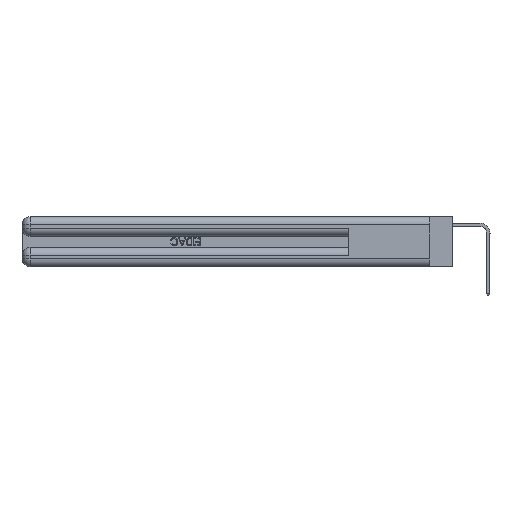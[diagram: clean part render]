
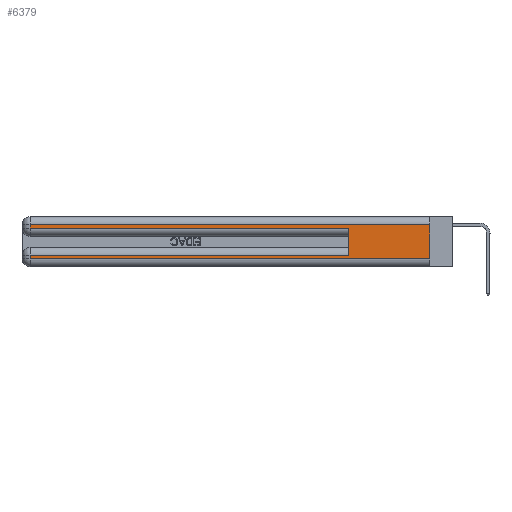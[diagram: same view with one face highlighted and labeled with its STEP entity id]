
A CAD part, left-side view. The second image highlights one B-rep face of the part: STEP entity #6379.
In plain terms, the highlighted planar face has unit normal (-1, 0, 0).
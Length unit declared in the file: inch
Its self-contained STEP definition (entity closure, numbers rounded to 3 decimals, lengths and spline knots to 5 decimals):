
#803 = CARTESIAN_POINT ( 'NONE',  ( 0., 0., 0.06 ) ) ;
#1108 = DIRECTION ( 'NONE',  ( 1., 0., 0. ) ) ;
#1264 = ORIENTED_EDGE ( 'NONE', *, *, #27751, .T. ) ;
#1280 = CARTESIAN_POINT ( 'NONE',  ( 0., 0., 0.085 ) ) ;
#1477 = CARTESIAN_POINT ( 'NONE',  ( 0., 0., 0.31 ) ) ;
#1805 = VERTEX_POINT ( 'NONE', #10659 ) ;
#2046 = VECTOR ( 'NONE', #2947, 39.37008 ) ;
#2652 = VECTOR ( 'NONE', #3811, 39.37008 ) ;
#2755 = EDGE_CURVE ( 'NONE', #1805, #22360, #28790, .T. ) ;
#2947 = DIRECTION ( 'NONE',  ( 0., -1., 0. ) ) ;
#3811 = DIRECTION ( 'NONE',  ( 0., 1., 0. ) ) ;
#4373 = ORIENTED_EDGE ( 'NONE', *, *, #18867, .F. ) ;
#4501 = ORIENTED_EDGE ( 'NONE', *, *, #19340, .T. ) ;
#4891 = DIRECTION ( 'NONE',  ( 0., 0., -1. ) ) ;
#5882 = LINE ( 'NONE', #19683, #18463 ) ;
#6379 = ADVANCED_FACE ( 'NONE', ( #28325 ), #21110, .F. ) ;
#6913 = ORIENTED_EDGE ( 'NONE', *, *, #18565, .T. ) ;
#7429 = CARTESIAN_POINT ( 'NONE',  ( 0., 2.94, 0.37 ) ) ;
#7513 = VECTOR ( 'NONE', #14542, 39.37008 ) ;
#7570 = ORIENTED_EDGE ( 'NONE', *, *, #12561, .F. ) ;
#8049 = VECTOR ( 'NONE', #4891, 39.37008 ) ;
#9258 = CARTESIAN_POINT ( 'NONE',  ( 0., 0.6, 0.085 ) ) ;
#9781 = EDGE_CURVE ( 'NONE', #11897, #27808, #30049, .T. ) ;
#10478 = DIRECTION ( 'NONE',  ( 0., 0., -1. ) ) ;
#10659 = CARTESIAN_POINT ( 'NONE',  ( 0., 2.94, 0.085 ) ) ;
#11897 = VERTEX_POINT ( 'NONE', #15726 ) ;
#12457 = VERTEX_POINT ( 'NONE', #9258 ) ;
#12561 = EDGE_CURVE ( 'NONE', #19216, #31814, #5882, .T. ) ;
#14406 = VECTOR ( 'NONE', #10478, 39.37008 ) ;
#14542 = DIRECTION ( 'NONE',  ( 0., 1., 0. ) ) ;
#14959 = LINE ( 'NONE', #24525, #7513 ) ;
#15470 = CARTESIAN_POINT ( 'NONE',  ( 0., 0., 0.06 ) ) ;
#15726 = CARTESIAN_POINT ( 'NONE',  ( 0., 2.94, 0.285 ) ) ;
#15993 = CARTESIAN_POINT ( 'NONE',  ( 0., 2.94, 0.06 ) ) ;
#17587 = VECTOR ( 'NONE', #32317, 39.37008 ) ;
#18463 = VECTOR ( 'NONE', #22222, 39.37008 ) ;
#18565 = EDGE_CURVE ( 'NONE', #22360, #31814, #22096, .T. ) ;
#18676 = DIRECTION ( 'NONE',  ( 0., 0., -1. ) ) ;
#18867 = EDGE_CURVE ( 'NONE', #12457, #27808, #26753, .T. ) ;
#19216 = VERTEX_POINT ( 'NONE', #1477 ) ;
#19340 = EDGE_CURVE ( 'NONE', #19216, #24897, #14959, .T. ) ;
#19683 = CARTESIAN_POINT ( 'NONE',  ( 0., 0., 0.37 ) ) ;
#21110 = PLANE ( 'NONE',  #25743 ) ;
#22096 = LINE ( 'NONE', #15470, #2046 ) ;
#22222 = DIRECTION ( 'NONE',  ( 0., 0., -1. ) ) ;
#22360 = VERTEX_POINT ( 'NONE', #15993 ) ;
#22440 = EDGE_LOOP ( 'NONE', ( #7570, #4501, #1264, #24228, #4373, #30800, #30573, #6913 ) ) ;
#22497 = DIRECTION ( 'NONE',  ( 0., 0., 1. ) ) ;
#22991 = CARTESIAN_POINT ( 'NONE',  ( 0., 2.94, 0.37 ) ) ;
#24228 = ORIENTED_EDGE ( 'NONE', *, *, #9781, .T. ) ;
#24525 = CARTESIAN_POINT ( 'NONE',  ( 0., 0., 0.31 ) ) ;
#24861 = CARTESIAN_POINT ( 'NONE',  ( 0., 0., 0.285 ) ) ;
#24897 = VERTEX_POINT ( 'NONE', #28374 ) ;
#25608 = CARTESIAN_POINT ( 'NONE',  ( 0., 0.6, 0.285 ) ) ;
#25743 = AXIS2_PLACEMENT_3D ( 'NONE', #31086, #1108, #18676 ) ;
#25965 = VECTOR ( 'NONE', #22497, 39.37008 ) ;
#26753 = LINE ( 'NONE', #29857, #25965 ) ;
#27751 = EDGE_CURVE ( 'NONE', #24897, #11897, #28472, .T. ) ;
#27808 = VERTEX_POINT ( 'NONE', #25608 ) ;
#28325 = FACE_OUTER_BOUND ( 'NONE', #22440, .T. ) ;
#28374 = CARTESIAN_POINT ( 'NONE',  ( 0., 2.94, 0.31 ) ) ;
#28472 = LINE ( 'NONE', #22991, #14406 ) ;
#28790 = LINE ( 'NONE', #7429, #8049 ) ;
#29261 = LINE ( 'NONE', #1280, #2652 ) ;
#29857 = CARTESIAN_POINT ( 'NONE',  ( 0., 0.6, 0.145 ) ) ;
#30049 = LINE ( 'NONE', #24861, #17587 ) ;
#30573 = ORIENTED_EDGE ( 'NONE', *, *, #2755, .T. ) ;
#30800 = ORIENTED_EDGE ( 'NONE', *, *, #31203, .T. ) ;
#31086 = CARTESIAN_POINT ( 'NONE',  ( 0., 0., 0.37 ) ) ;
#31203 = EDGE_CURVE ( 'NONE', #12457, #1805, #29261, .T. ) ;
#31814 = VERTEX_POINT ( 'NONE', #803 ) ;
#32317 = DIRECTION ( 'NONE',  ( 0., -1., 0. ) ) ;
